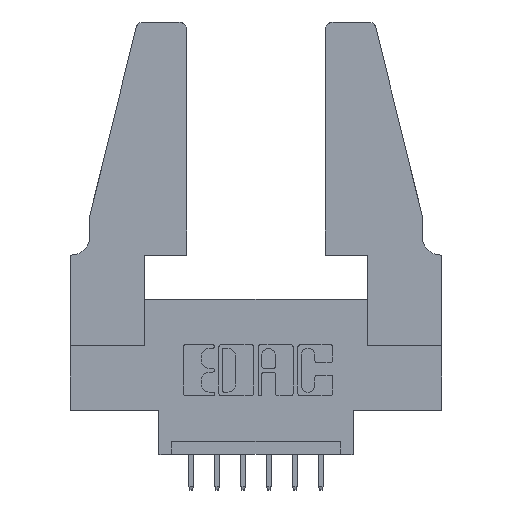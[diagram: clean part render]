
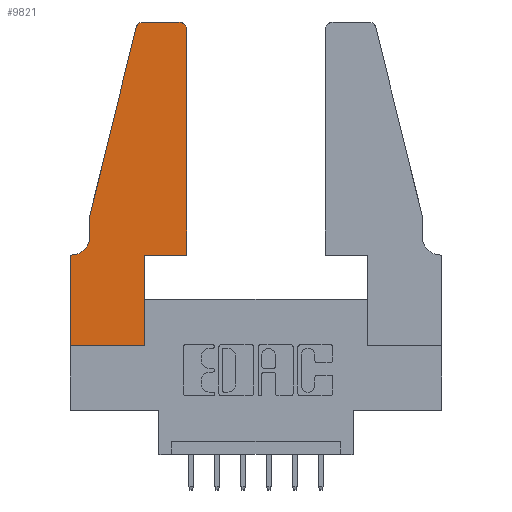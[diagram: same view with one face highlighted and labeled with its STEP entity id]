
A CAD part, top view. The second image highlights one B-rep face of the part: STEP entity #9821.
In plain terms, the highlighted planar face has unit normal (0, 0, 1).
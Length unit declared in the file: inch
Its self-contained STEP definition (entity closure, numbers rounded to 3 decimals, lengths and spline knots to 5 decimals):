
#230 = CARTESIAN_POINT ( 'NONE',  ( 0., 0.35, 0.37 ) ) ;
#582 = AXIS2_PLACEMENT_3D ( 'NONE', #7962, #2649, #668 ) ;
#606 = DIRECTION ( 'NONE',  ( 1., 0., 0. ) ) ;
#638 = LINE ( 'NONE', #700, #2511 ) ;
#668 = DIRECTION ( 'NONE',  ( -1., 0., 0. ) ) ;
#673 = VECTOR ( 'NONE', #6775, 39.37008 ) ;
#700 = CARTESIAN_POINT ( 'NONE',  ( 0.4505, 0.35, 0.37 ) ) ;
#869 = CARTESIAN_POINT ( 'NONE',  ( 0.4505, 0.35, 0.37 ) ) ;
#965 = VECTOR ( 'NONE', #2275, 39.37008 ) ;
#1149 = EDGE_CURVE ( 'NONE', #11231, #5869, #6892, .T. ) ;
#1452 = DIRECTION ( 'NONE',  ( 1., 0., 0. ) ) ;
#1506 = DIRECTION ( 'NONE',  ( 0., 0., 1. ) ) ;
#1637 = CARTESIAN_POINT ( 'NONE',  ( 0.2865, 0.35, 0.37 ) ) ;
#1802 = DIRECTION ( 'NONE',  ( 1., 0., 0. ) ) ;
#1946 = CIRCLE ( 'NONE', #5542, 0.03 ) ;
#2081 = EDGE_CURVE ( 'NONE', #3053, #9986, #7256, .T. ) ;
#2234 = ORIENTED_EDGE ( 'NONE', *, *, #8128, .T. ) ;
#2271 = ORIENTED_EDGE ( 'NONE', *, *, #10814, .T. ) ;
#2275 = DIRECTION ( 'NONE',  ( 1., 0., 0. ) ) ;
#2278 = DIRECTION ( 'NONE',  ( 1., 0., 0. ) ) ;
#2356 = DIRECTION ( 'NONE',  ( 0., -1., 0. ) ) ;
#2397 = CARTESIAN_POINT ( 'NONE',  ( 0.2865, 0.35, 0.37 ) ) ;
#2403 = VECTOR ( 'NONE', #2278, 39.37008 ) ;
#2423 = CARTESIAN_POINT ( 'NONE',  ( 0., 0., 0.37 ) ) ;
#2511 = VECTOR ( 'NONE', #5829, 39.37008 ) ;
#2649 = DIRECTION ( 'NONE',  ( 0., 0., -1. ) ) ;
#2652 = DIRECTION ( 'NONE',  ( 0., 0., 1. ) ) ;
#3053 = VERTEX_POINT ( 'NONE', #11355 ) ;
#3136 = CARTESIAN_POINT ( 'NONE',  ( 0.0755, 0.42, 0.37 ) ) ;
#3141 = AXIS2_PLACEMENT_3D ( 'NONE', #7015, #1506, #1452 ) ;
#3276 = EDGE_CURVE ( 'NONE', #4256, #4097, #7153, .T. ) ;
#3311 = CARTESIAN_POINT ( 'NONE',  ( 0.25487, 1.22718, 0.37 ) ) ;
#3423 = DIRECTION ( 'NONE',  ( 0., 0., 1. ) ) ;
#3551 = CARTESIAN_POINT ( 'NONE',  ( 0.4505, 1.22, 0.37 ) ) ;
#3578 = VERTEX_POINT ( 'NONE', #3136 ) ;
#3682 = CARTESIAN_POINT ( 'NONE',  ( 0.284, 1.25, 0.37 ) ) ;
#4005 = ORIENTED_EDGE ( 'NONE', *, *, #4038, .T. ) ;
#4038 = EDGE_CURVE ( 'NONE', #5477, #4256, #6882, .T. ) ;
#4088 = CARTESIAN_POINT ( 'NONE',  ( 0., 0., 0.37 ) ) ;
#4097 = VERTEX_POINT ( 'NONE', #2397 ) ;
#4133 = LINE ( 'NONE', #2423, #9217 ) ;
#4223 = ORIENTED_EDGE ( 'NONE', *, *, #1149, .T. ) ;
#4256 = VERTEX_POINT ( 'NONE', #10212 ) ;
#4356 = CARTESIAN_POINT ( 'NONE',  ( 0.4205, 1.22, 0.37 ) ) ;
#4378 = CARTESIAN_POINT ( 'NONE',  ( 0.4505, 0.35, 0.37 ) ) ;
#4412 = VECTOR ( 'NONE', #6482, 39.37008 ) ;
#4639 = DIRECTION ( 'NONE',  ( -1., 0., 0. ) ) ;
#4641 = EDGE_CURVE ( 'NONE', #11458, #3578, #4928, .T. ) ;
#4709 = LINE ( 'NONE', #10972, #4412 ) ;
#4928 = LINE ( 'NONE', #8548, #8257 ) ;
#4960 = VECTOR ( 'NONE', #4639, 39.37008 ) ;
#5129 = VERTEX_POINT ( 'NONE', #869 ) ;
#5234 = VECTOR ( 'NONE', #6245, 39.37008 ) ;
#5477 = VERTEX_POINT ( 'NONE', #4088 ) ;
#5500 = CARTESIAN_POINT ( 'NONE',  ( 0.0755, 0.5, 0.37 ) ) ;
#5542 = AXIS2_PLACEMENT_3D ( 'NONE', #4356, #3423, #1802 ) ;
#5583 = ORIENTED_EDGE ( 'NONE', *, *, #5849, .T. ) ;
#5612 = ORIENTED_EDGE ( 'NONE', *, *, #2081, .T. ) ;
#5649 = CARTESIAN_POINT ( 'NONE',  ( 0.4205, 1.25, 0.37 ) ) ;
#5655 = ORIENTED_EDGE ( 'NONE', *, *, #4641, .T. ) ;
#5829 = DIRECTION ( 'NONE',  ( 0., 1., 0. ) ) ;
#5849 = EDGE_CURVE ( 'NONE', #9986, #5477, #4133, .T. ) ;
#5869 = VERTEX_POINT ( 'NONE', #3311 ) ;
#6080 = ORIENTED_EDGE ( 'NONE', *, *, #8117, .T. ) ;
#6245 = DIRECTION ( 'NONE',  ( 0., 1., 0. ) ) ;
#6323 = ORIENTED_EDGE ( 'NONE', *, *, #10921, .T. ) ;
#6482 = DIRECTION ( 'NONE',  ( -0.239, -0.971, 0. ) ) ;
#6565 = ORIENTED_EDGE ( 'NONE', *, *, #3276, .T. ) ;
#6775 = DIRECTION ( 'NONE',  ( -1., 0., 0. ) ) ;
#6882 = LINE ( 'NONE', #7605, #2403 ) ;
#6892 = CIRCLE ( 'NONE', #3141, 0.03 ) ;
#7014 = PLANE ( 'NONE',  #7990 ) ;
#7015 = CARTESIAN_POINT ( 'NONE',  ( 0.284, 1.22, 0.37 ) ) ;
#7153 = LINE ( 'NONE', #1637, #5234 ) ;
#7159 = EDGE_LOOP ( 'NONE', ( #6080, #4223, #6323, #5655, #11298, #5612, #5583, #4005, #6565, #2234, #9282, #2271 ) ) ;
#7256 = LINE ( 'NONE', #9496, #673 ) ;
#7547 = DIRECTION ( 'NONE',  ( 0., -1., 0. ) ) ;
#7605 = CARTESIAN_POINT ( 'NONE',  ( 0., 0., 0.37 ) ) ;
#7962 = CARTESIAN_POINT ( 'NONE',  ( 0.0055, 0.42, 0.37 ) ) ;
#7990 = AXIS2_PLACEMENT_3D ( 'NONE', #10687, #2652, #606 ) ;
#8117 = EDGE_CURVE ( 'NONE', #9935, #11231, #10202, .T. ) ;
#8128 = EDGE_CURVE ( 'NONE', #4097, #5129, #10374, .T. ) ;
#8157 = EDGE_CURVE ( 'NONE', #5129, #10651, #638, .T. ) ;
#8257 = VECTOR ( 'NONE', #7547, 39.37008 ) ;
#8548 = CARTESIAN_POINT ( 'NONE',  ( 0.0755, 0.5, 0.37 ) ) ;
#9217 = VECTOR ( 'NONE', #2356, 39.37008 ) ;
#9282 = ORIENTED_EDGE ( 'NONE', *, *, #8157, .T. ) ;
#9455 = EDGE_CURVE ( 'NONE', #3578, #3053, #10808, .T. ) ;
#9496 = CARTESIAN_POINT ( 'NONE',  ( 0.0755, 0.35, 0.37 ) ) ;
#9743 = FACE_OUTER_BOUND ( 'NONE', #7159, .T. ) ;
#9821 = ADVANCED_FACE ( 'NONE', ( #9743 ), #7014, .T. ) ;
#9935 = VERTEX_POINT ( 'NONE', #5649 ) ;
#9986 = VERTEX_POINT ( 'NONE', #230 ) ;
#10202 = LINE ( 'NONE', #11026, #4960 ) ;
#10212 = CARTESIAN_POINT ( 'NONE',  ( 0.2865, 0., 0.37 ) ) ;
#10374 = LINE ( 'NONE', #4378, #965 ) ;
#10651 = VERTEX_POINT ( 'NONE', #3551 ) ;
#10687 = CARTESIAN_POINT ( 'NONE',  ( 0., 0.35, 0.37 ) ) ;
#10808 = CIRCLE ( 'NONE', #582, 0.07 ) ;
#10814 = EDGE_CURVE ( 'NONE', #10651, #9935, #1946, .T. ) ;
#10921 = EDGE_CURVE ( 'NONE', #5869, #11458, #4709, .T. ) ;
#10972 = CARTESIAN_POINT ( 'NONE',  ( 0.0755, 0.5, 0.37 ) ) ;
#11026 = CARTESIAN_POINT ( 'NONE',  ( 0.2605, 1.25, 0.37 ) ) ;
#11231 = VERTEX_POINT ( 'NONE', #3682 ) ;
#11298 = ORIENTED_EDGE ( 'NONE', *, *, #9455, .T. ) ;
#11355 = CARTESIAN_POINT ( 'NONE',  ( 0.0055, 0.35, 0.37 ) ) ;
#11458 = VERTEX_POINT ( 'NONE', #5500 ) ;
